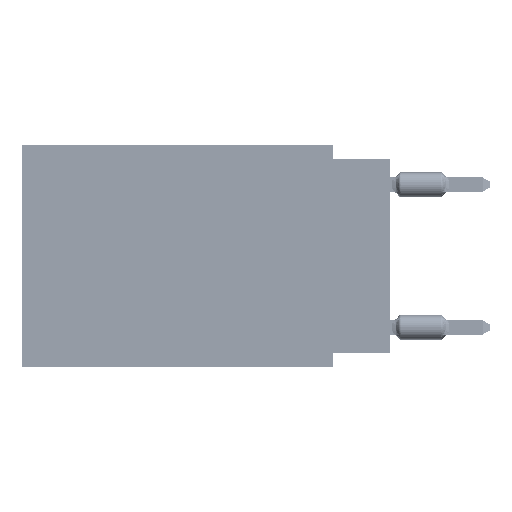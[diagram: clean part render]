
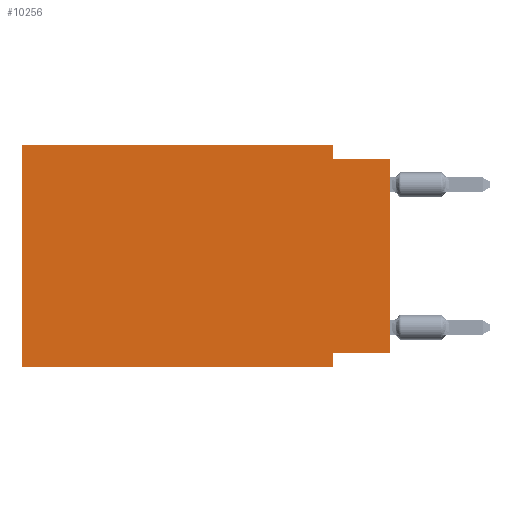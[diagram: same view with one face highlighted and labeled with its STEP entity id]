
A CAD part, left-side view. The second image highlights one B-rep face of the part: STEP entity #10256.
In plain terms, the highlighted planar face has unit normal (-1, 0, 0).
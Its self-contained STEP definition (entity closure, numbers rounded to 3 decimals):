
#1550 = CARTESIAN_POINT ( 'NONE',  ( 0., 0., -0.635 ) ) ;
#6858 = PLANE ( 'NONE',  #8511 ) ;
#8511 = AXIS2_PLACEMENT_3D ( 'NONE', #24306, #46458, #23583 ) ;
#8579 = LINE ( 'NONE', #19484, #18039 ) ;
#10256 = ADVANCED_FACE ( 'NONE', ( #56646 ), #6858, .F. ) ;
#10425 = LINE ( 'NONE', #27153, #67936 ) ;
#11032 = VECTOR ( 'NONE', #58698, 1000. ) ;
#11132 = LINE ( 'NONE', #1550, #66685 ) ;
#11408 = DIRECTION ( 'NONE',  ( 0., -1., 0. ) ) ;
#11901 = VECTOR ( 'NONE', #16767, 1000. ) ;
#12497 = EDGE_CURVE ( 'NONE', #55264, #69102, #17128, .T. ) ;
#13981 = CARTESIAN_POINT ( 'NONE',  ( 0., 2.54, -9.906 ) ) ;
#15804 = EDGE_LOOP ( 'NONE', ( #37269, #56328, #27979, #26922, #69990, #16370, #41727, #18287 ) ) ;
#16370 = ORIENTED_EDGE ( 'NONE', *, *, #43743, .T. ) ;
#16767 = DIRECTION ( 'NONE',  ( 0., 0., -1. ) ) ;
#17128 = LINE ( 'NONE', #55288, #11901 ) ;
#17250 = EDGE_CURVE ( 'NONE', #70282, #69878, #20901, .T. ) ;
#17471 = DIRECTION ( 'NONE',  ( 0., 0., 1. ) ) ;
#17571 = LINE ( 'NONE', #28837, #19926 ) ;
#18039 = VECTOR ( 'NONE', #26380, 1000. ) ;
#18287 = ORIENTED_EDGE ( 'NONE', *, *, #17250, .F. ) ;
#19484 = CARTESIAN_POINT ( 'NONE',  ( 0., 16.383, 0. ) ) ;
#19620 = CARTESIAN_POINT ( 'NONE',  ( 0., 16.383, 0. ) ) ;
#19926 = VECTOR ( 'NONE', #11408, 1000. ) ;
#20901 = LINE ( 'NONE', #48857, #25536 ) ;
#23048 = VERTEX_POINT ( 'NONE', #27029 ) ;
#23583 = DIRECTION ( 'NONE',  ( 0., 0., -1. ) ) ;
#24306 = CARTESIAN_POINT ( 'NONE',  ( 0., 16.383, 0. ) ) ;
#25536 = VECTOR ( 'NONE', #48164, 1000. ) ;
#25890 = CARTESIAN_POINT ( 'NONE',  ( 0., 2.54, 0. ) ) ;
#26380 = DIRECTION ( 'NONE',  ( 0., 0., 1. ) ) ;
#26922 = ORIENTED_EDGE ( 'NONE', *, *, #67954, .F. ) ;
#27029 = CARTESIAN_POINT ( 'NONE',  ( 0., 16.383, -9.906 ) ) ;
#27153 = CARTESIAN_POINT ( 'NONE',  ( 0., 16.383, 0. ) ) ;
#27979 = ORIENTED_EDGE ( 'NONE', *, *, #12497, .F. ) ;
#28739 = CARTESIAN_POINT ( 'NONE',  ( 0., 0., 0. ) ) ;
#28837 = CARTESIAN_POINT ( 'NONE',  ( 0., 16.383, -9.906 ) ) ;
#32846 = EDGE_CURVE ( 'NONE', #23048, #42680, #8579, .T. ) ;
#34905 = LINE ( 'NONE', #28739, #58399 ) ;
#37269 = ORIENTED_EDGE ( 'NONE', *, *, #62621, .T. ) ;
#37448 = CARTESIAN_POINT ( 'NONE',  ( 0., 2.54, -0.635 ) ) ;
#41727 = ORIENTED_EDGE ( 'NONE', *, *, #66976, .F. ) ;
#42201 = VERTEX_POINT ( 'NONE', #13981 ) ;
#42680 = VERTEX_POINT ( 'NONE', #19620 ) ;
#43047 = LINE ( 'NONE', #65210, #11032 ) ;
#43743 = EDGE_CURVE ( 'NONE', #23048, #42201, #17571, .T. ) ;
#44203 = DIRECTION ( 'NONE',  ( 0., -1., 0. ) ) ;
#46458 = DIRECTION ( 'NONE',  ( 1., 0., 0. ) ) ;
#48164 = DIRECTION ( 'NONE',  ( 0., 1., 0. ) ) ;
#48857 = CARTESIAN_POINT ( 'NONE',  ( 0., 0., -9.271 ) ) ;
#55082 = EDGE_CURVE ( 'NONE', #69102, #65726, #11132, .T. ) ;
#55264 = VERTEX_POINT ( 'NONE', #25890 ) ;
#55288 = CARTESIAN_POINT ( 'NONE',  ( 0., 2.54, 0. ) ) ;
#56328 = ORIENTED_EDGE ( 'NONE', *, *, #55082, .F. ) ;
#56646 = FACE_OUTER_BOUND ( 'NONE', #15804, .T. ) ;
#58399 = VECTOR ( 'NONE', #17471, 1000. ) ;
#58698 = DIRECTION ( 'NONE',  ( 0., 0., -1. ) ) ;
#62621 = EDGE_CURVE ( 'NONE', #70282, #65726, #34905, .T. ) ;
#63775 = CARTESIAN_POINT ( 'NONE',  ( 0., 0., -0.635 ) ) ;
#65210 = CARTESIAN_POINT ( 'NONE',  ( 0., 2.54, -9.906 ) ) ;
#65661 = DIRECTION ( 'NONE',  ( 0., -1., 0. ) ) ;
#65726 = VERTEX_POINT ( 'NONE', #63775 ) ;
#66685 = VECTOR ( 'NONE', #65661, 1000. ) ;
#66976 = EDGE_CURVE ( 'NONE', #69878, #42201, #43047, .T. ) ;
#67936 = VECTOR ( 'NONE', #44203, 1000. ) ;
#67954 = EDGE_CURVE ( 'NONE', #42680, #55264, #10425, .T. ) ;
#69102 = VERTEX_POINT ( 'NONE', #37448 ) ;
#69739 = CARTESIAN_POINT ( 'NONE',  ( 0., 2.54, -9.271 ) ) ;
#69878 = VERTEX_POINT ( 'NONE', #69739 ) ;
#69990 = ORIENTED_EDGE ( 'NONE', *, *, #32846, .F. ) ;
#70282 = VERTEX_POINT ( 'NONE', #71351 ) ;
#71351 = CARTESIAN_POINT ( 'NONE',  ( 0., 0., -9.271 ) ) ;
